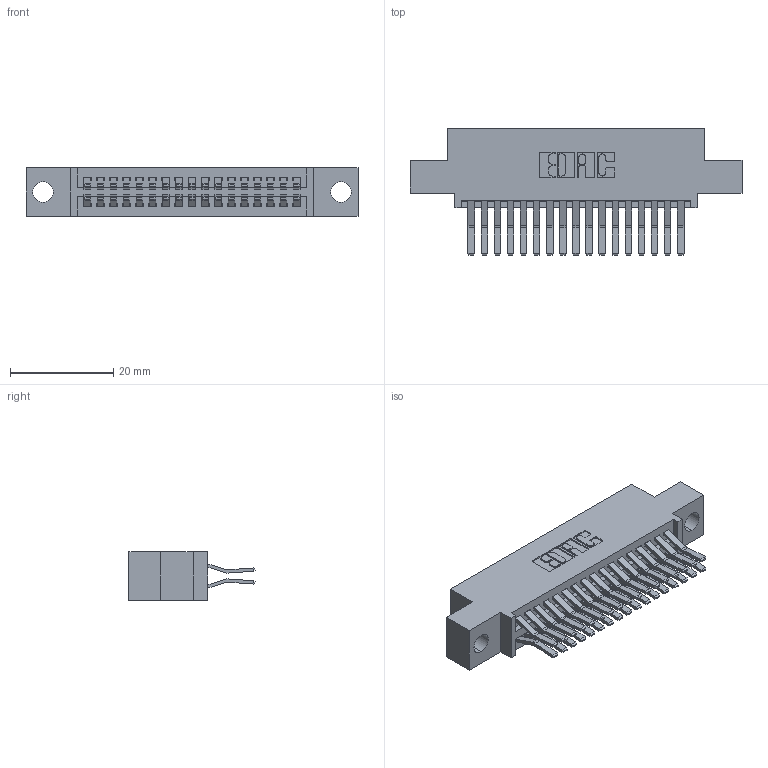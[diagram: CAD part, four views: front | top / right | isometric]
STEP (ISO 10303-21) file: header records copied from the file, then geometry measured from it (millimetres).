
FILE_DESCRIPTION (( 'STEP AP203' ), '1' );
FILE_NAME ('395-034-560-504.STEP', '2021-06-16T21:00:16', ( '' ), ( '' ), 'SwSTEP 2.0', 'SolidWorks 2020', '' );
FILE_SCHEMA (( 'CONFIG_CONTROL_DESIGN' ));
Length unit declared in the file: inch
Products named in the file (3): 345-292-001_560 Tail; 345 Part_0.110 Offset - 0.156 Dia-TI; 395-034-560-504
Assembly tree (35 placements, depth 2):
  395-034-560-504
    345 Part_0.110 Offset - 0.156 Dia-TI
    345-292-001_560 Tail  x34
Bounding box: 64.39 x 24.45 x 9.4 mm (x, y, z)
Volume: 6066.3 mm3; surface area: 9000.4 mm2
Topology: 35 solids, 35 shells, 1912 faces, 5659 edges, 3726 vertices
Faces by surface type: plane 1220, cylinder 692
Entity records: 17343 total; most frequent: CARTESIAN_POINT 2938, ORIENTED_EDGE 2870, DIRECTION 2623, EDGE_CURVE 1435, VECTOR 1231, LINE 1231, VERTEX_POINT 954, AXIS2_PLACEMENT_3D 696
